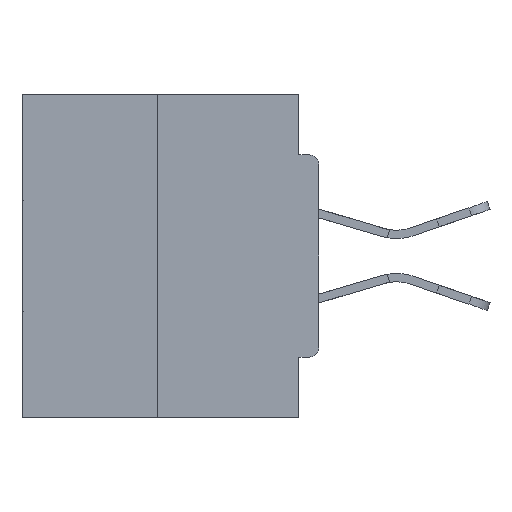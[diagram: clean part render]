
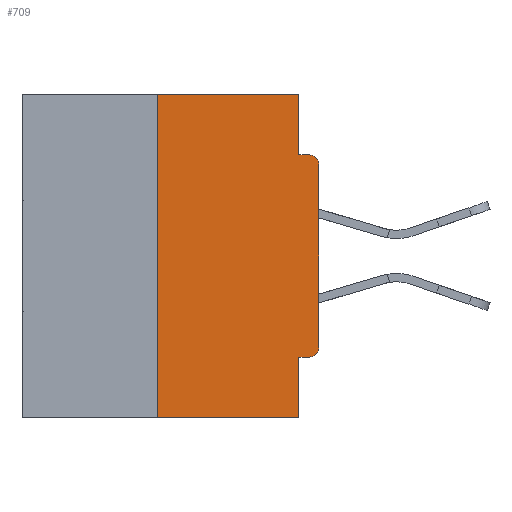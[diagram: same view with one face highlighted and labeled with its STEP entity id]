
A CAD part, left-side view. The second image highlights one B-rep face of the part: STEP entity #709.
In plain terms, the highlighted planar face has unit normal (-1, 0, 0).
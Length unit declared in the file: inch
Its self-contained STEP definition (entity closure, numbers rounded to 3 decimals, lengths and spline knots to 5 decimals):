
#704 = CARTESIAN_POINT ( 'NONE',  ( 0., 0., -0.0935 ) ) ;
#709 = ADVANCED_FACE ( 'NONE', ( #33083 ), #30855, .F. ) ;
#764 = DIRECTION ( 'NONE',  ( 0., -1., 0. ) ) ;
#1511 = EDGE_CURVE ( 'NONE', #18275, #23873, #7747, .T. ) ;
#1856 = DIRECTION ( 'NONE',  ( 0., 0., -1. ) ) ;
#2200 = AXIS2_PLACEMENT_3D ( 'NONE', #3351, #9651, #12291 ) ;
#2714 = ORIENTED_EDGE ( 'NONE', *, *, #25110, .T. ) ;
#3133 = LINE ( 'NONE', #20144, #34678 ) ;
#3351 = CARTESIAN_POINT ( 'NONE',  ( 0., 0.46, 0. ) ) ;
#3468 = CARTESIAN_POINT ( 'NONE',  ( 0., 0.25, 0. ) ) ;
#3587 = DIRECTION ( 'NONE',  ( 0., 0., 1. ) ) ;
#4806 = DIRECTION ( 'NONE',  ( -1., 0., 0. ) ) ;
#5054 = CIRCLE ( 'NONE', #12596, 0.015 ) ;
#5271 = ORIENTED_EDGE ( 'NONE', *, *, #18252, .F. ) ;
#6149 = CARTESIAN_POINT ( 'NONE',  ( 0., 0., -0.1085 ) ) ;
#6541 = CARTESIAN_POINT ( 'NONE',  ( 0., 0.031, 0. ) ) ;
#7551 = CARTESIAN_POINT ( 'NONE',  ( 0., 0., -0.4065 ) ) ;
#7747 = LINE ( 'NONE', #22622, #39291 ) ;
#8154 = VERTEX_POINT ( 'NONE', #26191 ) ;
#9651 = DIRECTION ( 'NONE',  ( 1., 0., 0. ) ) ;
#10109 = ORIENTED_EDGE ( 'NONE', *, *, #27720, .T. ) ;
#10216 = DIRECTION ( 'NONE',  ( 0., 0., -1. ) ) ;
#10241 = CARTESIAN_POINT ( 'NONE',  ( 0., 0.015, -0.0935 ) ) ;
#12291 = DIRECTION ( 'NONE',  ( 0., 0., -1. ) ) ;
#12596 = AXIS2_PLACEMENT_3D ( 'NONE', #35264, #4806, #1856 ) ;
#12848 = EDGE_CURVE ( 'NONE', #18321, #14084, #5054, .T. ) ;
#13666 = VECTOR ( 'NONE', #19145, 39.37008 ) ;
#13669 = DIRECTION ( 'NONE',  ( 0., -1., 0. ) ) ;
#13737 = EDGE_CURVE ( 'NONE', #15220, #8154, #14110, .T. ) ;
#14084 = VERTEX_POINT ( 'NONE', #21788 ) ;
#14110 = LINE ( 'NONE', #28500, #26501 ) ;
#14995 = VERTEX_POINT ( 'NONE', #3468 ) ;
#15220 = VERTEX_POINT ( 'NONE', #38014 ) ;
#15990 = VECTOR ( 'NONE', #3587, 39.37008 ) ;
#17200 = ORIENTED_EDGE ( 'NONE', *, *, #19019, .F. ) ;
#17752 = CARTESIAN_POINT ( 'NONE',  ( 0., 0.031, -0.0935 ) ) ;
#17776 = DIRECTION ( 'NONE',  ( 0., -1., 0. ) ) ;
#17978 = EDGE_CURVE ( 'NONE', #18345, #14995, #33243, .T. ) ;
#18252 = EDGE_CURVE ( 'NONE', #14995, #18275, #3133, .T. ) ;
#18275 = VERTEX_POINT ( 'NONE', #6541 ) ;
#18321 = VERTEX_POINT ( 'NONE', #24344 ) ;
#18345 = VERTEX_POINT ( 'NONE', #38304 ) ;
#18699 = CIRCLE ( 'NONE', #22155, 0.015 ) ;
#18880 = ORIENTED_EDGE ( 'NONE', *, *, #1511, .F. ) ;
#19015 = CARTESIAN_POINT ( 'NONE',  ( 0., 0.25, 0. ) ) ;
#19019 = EDGE_CURVE ( 'NONE', #23873, #34756, #21682, .T. ) ;
#19079 = EDGE_CURVE ( 'NONE', #14084, #33839, #31263, .T. ) ;
#19145 = DIRECTION ( 'NONE',  ( 0., 0., 1. ) ) ;
#20144 = CARTESIAN_POINT ( 'NONE',  ( 0., 0.46, 0. ) ) ;
#21682 = LINE ( 'NONE', #704, #37495 ) ;
#21788 = CARTESIAN_POINT ( 'NONE',  ( 0., 0., -0.3915 ) ) ;
#21953 = ORIENTED_EDGE ( 'NONE', *, *, #29219, .F. ) ;
#22155 = AXIS2_PLACEMENT_3D ( 'NONE', #22379, #25143, #34405 ) ;
#22379 = CARTESIAN_POINT ( 'NONE',  ( 0., 0.015, -0.1085 ) ) ;
#22622 = CARTESIAN_POINT ( 'NONE',  ( 0., 0.031, 0. ) ) ;
#23171 = DIRECTION ( 'NONE',  ( 0., 1., 0. ) ) ;
#23639 = VECTOR ( 'NONE', #23171, 39.37008 ) ;
#23873 = VERTEX_POINT ( 'NONE', #17752 ) ;
#24344 = CARTESIAN_POINT ( 'NONE',  ( 0., 0.015, -0.4065 ) ) ;
#25110 = EDGE_CURVE ( 'NONE', #33839, #34756, #18699, .T. ) ;
#25143 = DIRECTION ( 'NONE',  ( -1., 0., 0. ) ) ;
#26191 = CARTESIAN_POINT ( 'NONE',  ( 0., 0.031, -0.5 ) ) ;
#26438 = EDGE_LOOP ( 'NONE', ( #5271, #32409, #10109, #27123, #21953, #34175, #37017, #2714, #17200, #18880 ) ) ;
#26501 = VECTOR ( 'NONE', #37471, 39.37008 ) ;
#26965 = LINE ( 'NONE', #7551, #23639 ) ;
#27123 = ORIENTED_EDGE ( 'NONE', *, *, #13737, .F. ) ;
#27185 = VECTOR ( 'NONE', #13669, 39.37008 ) ;
#27720 = EDGE_CURVE ( 'NONE', #18345, #8154, #32502, .T. ) ;
#28500 = CARTESIAN_POINT ( 'NONE',  ( 0., 0.031, -0.5 ) ) ;
#29219 = EDGE_CURVE ( 'NONE', #18321, #15220, #26965, .T. ) ;
#30855 = PLANE ( 'NONE',  #2200 ) ;
#31263 = LINE ( 'NONE', #36585, #15990 ) ;
#31845 = CARTESIAN_POINT ( 'NONE',  ( 0., 0.46, -0.5 ) ) ;
#32409 = ORIENTED_EDGE ( 'NONE', *, *, #17978, .F. ) ;
#32502 = LINE ( 'NONE', #31845, #27185 ) ;
#33083 = FACE_OUTER_BOUND ( 'NONE', #26438, .T. ) ;
#33243 = LINE ( 'NONE', #19015, #13666 ) ;
#33839 = VERTEX_POINT ( 'NONE', #6149 ) ;
#34175 = ORIENTED_EDGE ( 'NONE', *, *, #12848, .T. ) ;
#34405 = DIRECTION ( 'NONE',  ( 0., 0., -1. ) ) ;
#34678 = VECTOR ( 'NONE', #764, 39.37008 ) ;
#34756 = VERTEX_POINT ( 'NONE', #10241 ) ;
#35264 = CARTESIAN_POINT ( 'NONE',  ( 0., 0.015, -0.3915 ) ) ;
#36585 = CARTESIAN_POINT ( 'NONE',  ( 0., 0., 0. ) ) ;
#37017 = ORIENTED_EDGE ( 'NONE', *, *, #19079, .T. ) ;
#37471 = DIRECTION ( 'NONE',  ( 0., 0., -1. ) ) ;
#37495 = VECTOR ( 'NONE', #17776, 39.37008 ) ;
#38014 = CARTESIAN_POINT ( 'NONE',  ( 0., 0.031, -0.4065 ) ) ;
#38304 = CARTESIAN_POINT ( 'NONE',  ( 0., 0.25, -0.5 ) ) ;
#39291 = VECTOR ( 'NONE', #10216, 39.37008 ) ;
